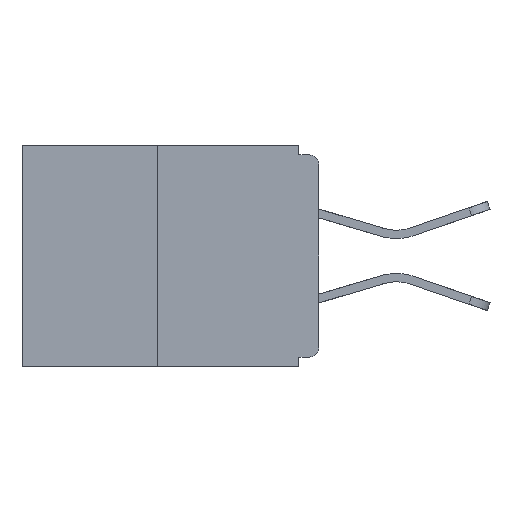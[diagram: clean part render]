
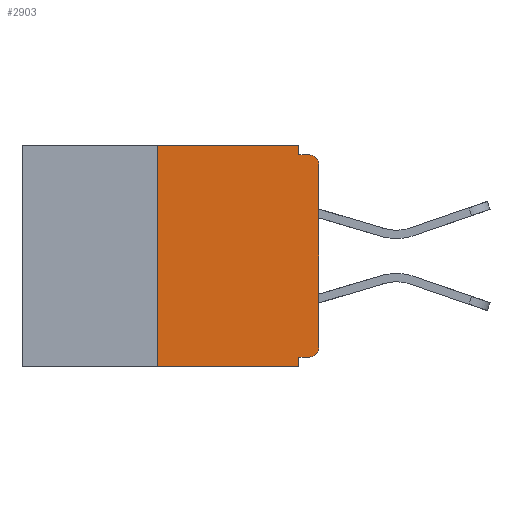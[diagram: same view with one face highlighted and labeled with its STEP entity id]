
A CAD part, left-side view. The second image highlights one B-rep face of the part: STEP entity #2903.
In plain terms, the highlighted planar face has unit normal (-1, 0, 0).
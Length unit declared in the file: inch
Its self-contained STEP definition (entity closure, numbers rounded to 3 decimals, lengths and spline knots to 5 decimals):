
#703 = ORIENTED_EDGE ( 'NONE', *, *, #4666, .T. ) ;
#916 = ORIENTED_EDGE ( 'NONE', *, *, #7599, .F. ) ;
#1526 = EDGE_CURVE ( 'NONE', #15730, #16945, #18392, .T. ) ;
#1587 = CIRCLE ( 'NONE', #9020, 0.015 ) ;
#1647 = EDGE_CURVE ( 'NONE', #6939, #19035, #5418, .T. ) ;
#2869 = DIRECTION ( 'NONE',  ( 0., 0., -1. ) ) ;
#2903 = ADVANCED_FACE ( 'NONE', ( #5022 ), #3889, .F. ) ;
#3106 = VERTEX_POINT ( 'NONE', #25056 ) ;
#3553 = VECTOR ( 'NONE', #15311, 39.37008 ) ;
#3673 = CARTESIAN_POINT ( 'NONE',  ( 0., 0.25, -0.343 ) ) ;
#3755 = LINE ( 'NONE', #14161, #4992 ) ;
#3868 = LINE ( 'NONE', #4386, #21534 ) ;
#3889 = PLANE ( 'NONE',  #16579 ) ;
#3975 = DIRECTION ( 'NONE',  ( 0., 0., 1. ) ) ;
#3978 = DIRECTION ( 'NONE',  ( 1., 0., 0. ) ) ;
#4386 = CARTESIAN_POINT ( 'NONE',  ( 0., 0.46, -0.343 ) ) ;
#4494 = VECTOR ( 'NONE', #2869, 39.37008 ) ;
#4594 = CARTESIAN_POINT ( 'NONE',  ( 0., 0.015, -0.03 ) ) ;
#4666 = EDGE_CURVE ( 'NONE', #21995, #22256, #3755, .T. ) ;
#4992 = VECTOR ( 'NONE', #26082, 39.37008 ) ;
#5022 = FACE_OUTER_BOUND ( 'NONE', #17168, .T. ) ;
#5365 = DIRECTION ( 'NONE',  ( 0., 0., -1. ) ) ;
#5418 = LINE ( 'NONE', #13956, #19016 ) ;
#5924 = DIRECTION ( 'NONE',  ( 0., 0., -1. ) ) ;
#6939 = VERTEX_POINT ( 'NONE', #3673 ) ;
#7484 = ORIENTED_EDGE ( 'NONE', *, *, #1647, .F. ) ;
#7599 = EDGE_CURVE ( 'NONE', #17471, #17013, #12131, .T. ) ;
#7772 = CARTESIAN_POINT ( 'NONE',  ( 0., 0.25, 0. ) ) ;
#8299 = DIRECTION ( 'NONE',  ( 0., -1., 0. ) ) ;
#8350 = DIRECTION ( 'NONE',  ( 0., 0., -1. ) ) ;
#9020 = AXIS2_PLACEMENT_3D ( 'NONE', #17388, #9383, #5365 ) ;
#9326 = DIRECTION ( 'NONE',  ( 0., -1., 0. ) ) ;
#9383 = DIRECTION ( 'NONE',  ( -1., 0., 0. ) ) ;
#9815 = CARTESIAN_POINT ( 'NONE',  ( 0., 0.46, 0. ) ) ;
#9849 = ORIENTED_EDGE ( 'NONE', *, *, #1526, .F. ) ;
#10566 = CARTESIAN_POINT ( 'NONE',  ( 0., 0., -0.03 ) ) ;
#10741 = CARTESIAN_POINT ( 'NONE',  ( 0., 0., -0.015 ) ) ;
#10876 = VECTOR ( 'NONE', #9326, 39.37008 ) ;
#11521 = AXIS2_PLACEMENT_3D ( 'NONE', #4594, #18715, #8350 ) ;
#11856 = DIRECTION ( 'NONE',  ( 0., 0., -1. ) ) ;
#12131 = LINE ( 'NONE', #10741, #15871 ) ;
#12364 = ORIENTED_EDGE ( 'NONE', *, *, #14378, .T. ) ;
#12610 = CARTESIAN_POINT ( 'NONE',  ( 0., 0.46, 0. ) ) ;
#12714 = LINE ( 'NONE', #23085, #4494 ) ;
#12763 = DIRECTION ( 'NONE',  ( 0., -1., 0. ) ) ;
#13164 = EDGE_CURVE ( 'NONE', #6939, #23699, #3868, .T. ) ;
#13545 = EDGE_CURVE ( 'NONE', #22256, #17013, #19953, .T. ) ;
#13956 = CARTESIAN_POINT ( 'NONE',  ( 0., 0.25, 0. ) ) ;
#14161 = CARTESIAN_POINT ( 'NONE',  ( 0., 0., 0. ) ) ;
#14378 = EDGE_CURVE ( 'NONE', #15730, #21995, #1587, .T. ) ;
#15311 = DIRECTION ( 'NONE',  ( 0., 1., 0. ) ) ;
#15730 = VERTEX_POINT ( 'NONE', #24728 ) ;
#15871 = VECTOR ( 'NONE', #12763, 39.37008 ) ;
#16579 = AXIS2_PLACEMENT_3D ( 'NONE', #9815, #3978, #5924 ) ;
#16791 = CARTESIAN_POINT ( 'NONE',  ( 0., 0.015, -0.015 ) ) ;
#16887 = CARTESIAN_POINT ( 'NONE',  ( 0., 0., -0.313 ) ) ;
#16945 = VERTEX_POINT ( 'NONE', #24836 ) ;
#17013 = VERTEX_POINT ( 'NONE', #16791 ) ;
#17168 = EDGE_LOOP ( 'NONE', ( #19461, #7484, #19843, #22162, #9849, #12364, #703, #17791, #916, #22840 ) ) ;
#17388 = CARTESIAN_POINT ( 'NONE',  ( 0., 0.015, -0.313 ) ) ;
#17431 = EDGE_CURVE ( 'NONE', #19035, #3106, #25073, .T. ) ;
#17471 = VERTEX_POINT ( 'NONE', #17655 ) ;
#17655 = CARTESIAN_POINT ( 'NONE',  ( 0., 0.031, -0.015 ) ) ;
#17791 = ORIENTED_EDGE ( 'NONE', *, *, #13545, .T. ) ;
#18392 = LINE ( 'NONE', #19580, #3553 ) ;
#18715 = DIRECTION ( 'NONE',  ( -1., 0., 0. ) ) ;
#19016 = VECTOR ( 'NONE', #3975, 39.37008 ) ;
#19035 = VERTEX_POINT ( 'NONE', #7772 ) ;
#19461 = ORIENTED_EDGE ( 'NONE', *, *, #17431, .F. ) ;
#19580 = CARTESIAN_POINT ( 'NONE',  ( 0., 0., -0.328 ) ) ;
#19843 = ORIENTED_EDGE ( 'NONE', *, *, #13164, .T. ) ;
#19953 = CIRCLE ( 'NONE', #11521, 0.015 ) ;
#21005 = VECTOR ( 'NONE', #11856, 39.37008 ) ;
#21534 = VECTOR ( 'NONE', #8299, 39.37008 ) ;
#21733 = CARTESIAN_POINT ( 'NONE',  ( 0., 0.031, 0. ) ) ;
#21995 = VERTEX_POINT ( 'NONE', #16887 ) ;
#22162 = ORIENTED_EDGE ( 'NONE', *, *, #25731, .F. ) ;
#22256 = VERTEX_POINT ( 'NONE', #10566 ) ;
#22840 = ORIENTED_EDGE ( 'NONE', *, *, #24134, .F. ) ;
#23085 = CARTESIAN_POINT ( 'NONE',  ( 0., 0.031, -0.343 ) ) ;
#23699 = VERTEX_POINT ( 'NONE', #24334 ) ;
#24134 = EDGE_CURVE ( 'NONE', #3106, #17471, #26078, .T. ) ;
#24334 = CARTESIAN_POINT ( 'NONE',  ( 0., 0.031, -0.343 ) ) ;
#24728 = CARTESIAN_POINT ( 'NONE',  ( 0., 0.015, -0.328 ) ) ;
#24836 = CARTESIAN_POINT ( 'NONE',  ( 0., 0.031, -0.328 ) ) ;
#25056 = CARTESIAN_POINT ( 'NONE',  ( 0., 0.031, 0. ) ) ;
#25073 = LINE ( 'NONE', #12610, #10876 ) ;
#25731 = EDGE_CURVE ( 'NONE', #16945, #23699, #12714, .T. ) ;
#26078 = LINE ( 'NONE', #21733, #21005 ) ;
#26082 = DIRECTION ( 'NONE',  ( 0., 0., 1. ) ) ;
